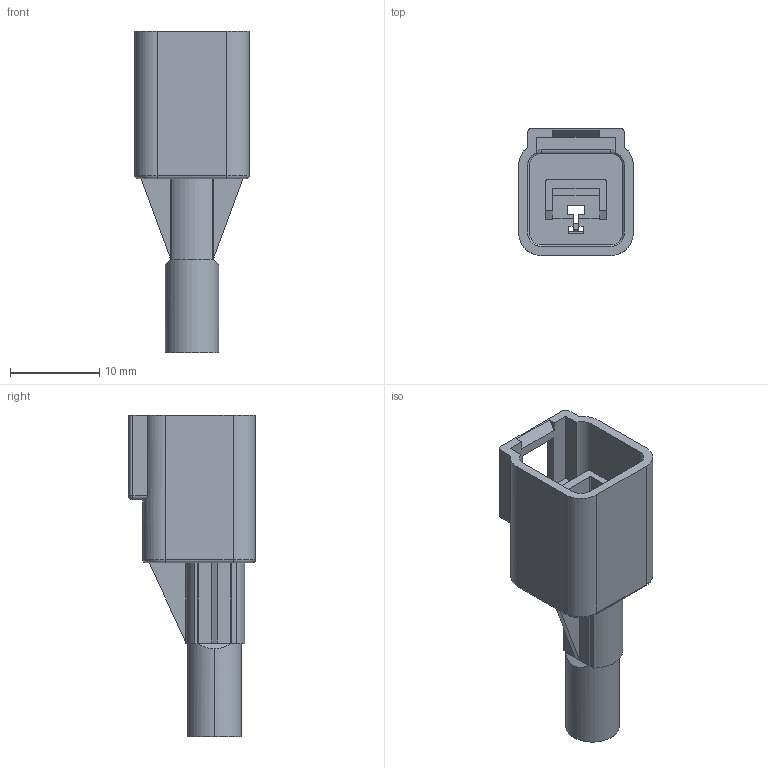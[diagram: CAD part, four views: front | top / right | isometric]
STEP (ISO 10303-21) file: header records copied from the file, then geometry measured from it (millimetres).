
FILE_DESCRIPTION (( 'STEP AP214' ), '1' );
FILE_NAME ('570-001-000-100.STEP', '2020-07-30T14:03:16', ( '' ), ( '' ), 'SwSTEP 2.0', 'SolidWorks 2020', '' );
FILE_SCHEMA (( 'AUTOMOTIVE_DESIGN' ));
Length unit declared in the file: millimetre
Products named in the file (1): 570-001-000-100
Bounding box: 12.8 x 14.2 x 36 mm (x, y, z)
Volume: 1424.8 mm3; surface area: 2771.1 mm2
Topology: 2 solids, 2 shells, 141 faces, 375 edges, 238 vertices
Faces by surface type: plane 97, cylinder 31, torus 6, cone 4, sphere 2, bspline 1
Entity records: 4378 total; most frequent: CARTESIAN_POINT 813, ORIENTED_EDGE 746, DIRECTION 717, EDGE_CURVE 373, VECTOR 281, LINE 281, VERTEX_POINT 238, AXIS2_PLACEMENT_3D 218
